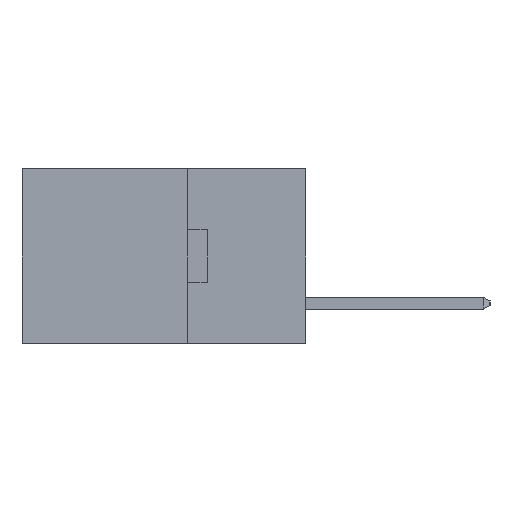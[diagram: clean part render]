
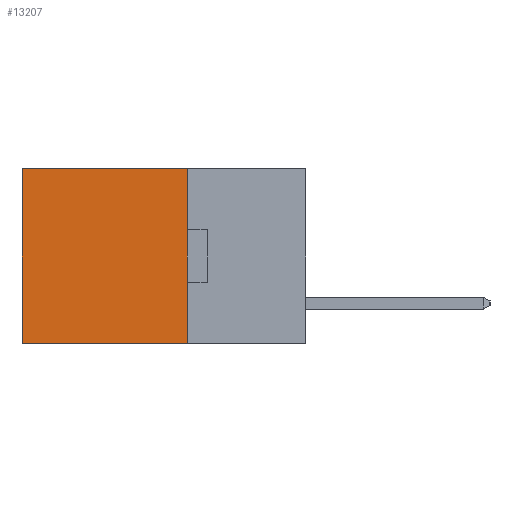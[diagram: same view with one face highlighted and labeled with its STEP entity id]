
A CAD part, left-side view. The second image highlights one B-rep face of the part: STEP entity #13207.
In plain terms, the highlighted planar face has unit normal (-1, 0, 0).
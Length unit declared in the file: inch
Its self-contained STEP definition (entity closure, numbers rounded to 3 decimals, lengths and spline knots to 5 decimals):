
#488 = CARTESIAN_POINT ( 'NONE',  ( 0.2615, 0.25, -0.37 ) ) ;
#3046 = ORIENTED_EDGE ( 'NONE', *, *, #21922, .F. ) ;
#3439 = VECTOR ( 'NONE', #17152, 39.37008 ) ;
#3635 = ORIENTED_EDGE ( 'NONE', *, *, #6014, .T. ) ;
#3835 = ORIENTED_EDGE ( 'NONE', *, *, #8130, .F. ) ;
#4251 = EDGE_CURVE ( 'NONE', #4500, #11862, #10820, .T. ) ;
#4500 = VERTEX_POINT ( 'NONE', #8690 ) ;
#6014 = EDGE_CURVE ( 'NONE', #11862, #12338, #14555, .T. ) ;
#7499 = CARTESIAN_POINT ( 'NONE',  ( 0.2615, 0.6, 0. ) ) ;
#8130 = EDGE_CURVE ( 'NONE', #11752, #12338, #8349, .T. ) ;
#8349 = LINE ( 'NONE', #488, #3439 ) ;
#8416 = FACE_OUTER_BOUND ( 'NONE', #11480, .T. ) ;
#8690 = CARTESIAN_POINT ( 'NONE',  ( 0.2615, 0.25, 0. ) ) ;
#9925 = ORIENTED_EDGE ( 'NONE', *, *, #4251, .T. ) ;
#10716 = DIRECTION ( 'NONE',  ( 1., 0., 0. ) ) ;
#10820 = LINE ( 'NONE', #18198, #21115 ) ;
#11480 = EDGE_LOOP ( 'NONE', ( #3635, #3835, #3046, #9925 ) ) ;
#11672 = AXIS2_PLACEMENT_3D ( 'NONE', #23064, #10716, #25119 ) ;
#11752 = VERTEX_POINT ( 'NONE', #19550 ) ;
#11862 = VERTEX_POINT ( 'NONE', #7499 ) ;
#12338 = VERTEX_POINT ( 'NONE', #21498 ) ;
#12711 = PLANE ( 'NONE',  #11672 ) ;
#12923 = DIRECTION ( 'NONE',  ( 0., 0., -1. ) ) ;
#13207 = ADVANCED_FACE ( 'NONE', ( #8416 ), #12711, .F. ) ;
#14078 = DIRECTION ( 'NONE',  ( 0., 1., 0. ) ) ;
#14555 = LINE ( 'NONE', #19031, #19378 ) ;
#17152 = DIRECTION ( 'NONE',  ( 0., 1., 0. ) ) ;
#17168 = CARTESIAN_POINT ( 'NONE',  ( 0.2615, 0.25, -0.37 ) ) ;
#18198 = CARTESIAN_POINT ( 'NONE',  ( 0.2615, 0.25, 0. ) ) ;
#19031 = CARTESIAN_POINT ( 'NONE',  ( 0.2615, 0.6, -0.37 ) ) ;
#19378 = VECTOR ( 'NONE', #12923, 39.37008 ) ;
#19550 = CARTESIAN_POINT ( 'NONE',  ( 0.2615, 0.25, -0.37 ) ) ;
#20300 = VECTOR ( 'NONE', #25439, 39.37008 ) ;
#21115 = VECTOR ( 'NONE', #14078, 39.37008 ) ;
#21498 = CARTESIAN_POINT ( 'NONE',  ( 0.2615, 0.6, -0.37 ) ) ;
#21922 = EDGE_CURVE ( 'NONE', #4500, #11752, #25767, .T. ) ;
#23064 = CARTESIAN_POINT ( 'NONE',  ( 0.2615, 0.25, -0.37 ) ) ;
#25119 = DIRECTION ( 'NONE',  ( 0., 0., -1. ) ) ;
#25439 = DIRECTION ( 'NONE',  ( 0., 0., -1. ) ) ;
#25767 = LINE ( 'NONE', #17168, #20300 ) ;
